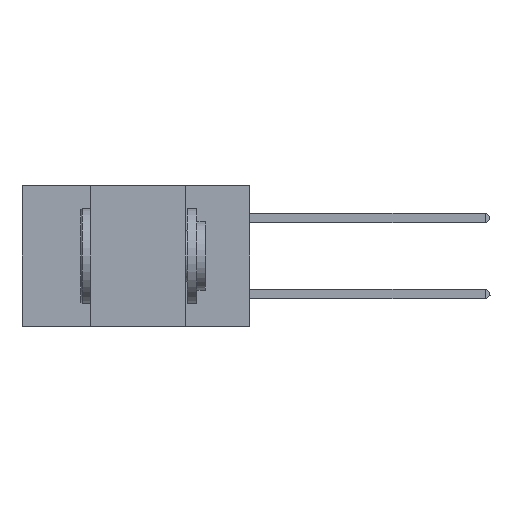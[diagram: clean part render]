
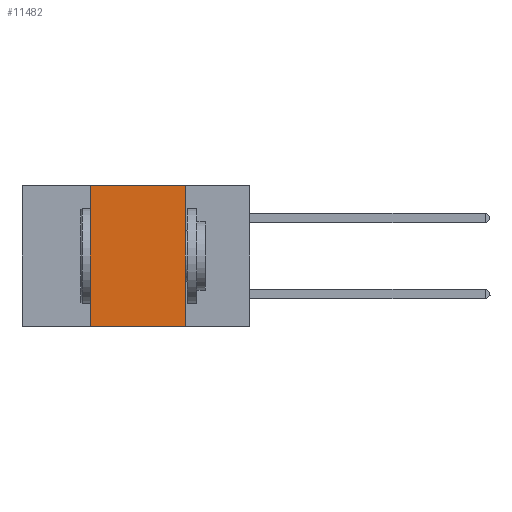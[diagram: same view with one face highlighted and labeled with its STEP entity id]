
A CAD part, left-side view. The second image highlights one B-rep face of the part: STEP entity #11482.
In plain terms, the highlighted planar face has unit normal (-1, 0, 0).
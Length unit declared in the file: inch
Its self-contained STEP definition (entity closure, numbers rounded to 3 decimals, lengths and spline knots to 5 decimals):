
#1263 = DIRECTION ( 'NONE',  ( 0., -1., 0. ) ) ;
#2690 = LINE ( 'NONE', #13811, #7510 ) ;
#3364 = ORIENTED_EDGE ( 'NONE', *, *, #7947, .F. ) ;
#3888 = VERTEX_POINT ( 'NONE', #11872 ) ;
#3892 = LINE ( 'NONE', #11522, #5864 ) ;
#4083 = LINE ( 'NONE', #10778, #4418 ) ;
#4418 = VECTOR ( 'NONE', #17061, 39.37008 ) ;
#5084 = EDGE_CURVE ( 'NONE', #7061, #24200, #3892, .T. ) ;
#5864 = VECTOR ( 'NONE', #1263, 39.37008 ) ;
#6577 = AXIS2_PLACEMENT_3D ( 'NONE', #9366, #25647, #23700 ) ;
#7061 = VERTEX_POINT ( 'NONE', #21695 ) ;
#7291 = ORIENTED_EDGE ( 'NONE', *, *, #5084, .T. ) ;
#7510 = VECTOR ( 'NONE', #16048, 39.37008 ) ;
#7820 = EDGE_CURVE ( 'NONE', #10284, #3888, #2690, .T. ) ;
#7947 = EDGE_CURVE ( 'NONE', #7061, #10284, #12019, .T. ) ;
#9285 = PLANE ( 'NONE',  #6577 ) ;
#9366 = CARTESIAN_POINT ( 'NONE',  ( 0., 0.6, 0. ) ) ;
#10284 = VERTEX_POINT ( 'NONE', #13207 ) ;
#10467 = ORIENTED_EDGE ( 'NONE', *, *, #7820, .F. ) ;
#10729 = EDGE_CURVE ( 'NONE', #3888, #24200, #4083, .T. ) ;
#10778 = CARTESIAN_POINT ( 'NONE',  ( 0., 0.17, 0. ) ) ;
#11482 = ADVANCED_FACE ( 'NONE', ( #15931 ), #9285, .F. ) ;
#11522 = CARTESIAN_POINT ( 'NONE',  ( 0., 0.6, -0.37 ) ) ;
#11872 = CARTESIAN_POINT ( 'NONE',  ( 0., 0.17, 0. ) ) ;
#12019 = LINE ( 'NONE', #14170, #20092 ) ;
#12387 = DIRECTION ( 'NONE',  ( 0., 0., 1. ) ) ;
#12633 = EDGE_LOOP ( 'NONE', ( #26309, #10467, #3364, #7291 ) ) ;
#13207 = CARTESIAN_POINT ( 'NONE',  ( 0., 0.42, 0. ) ) ;
#13811 = CARTESIAN_POINT ( 'NONE',  ( 0., 0.6, 0. ) ) ;
#14170 = CARTESIAN_POINT ( 'NONE',  ( 0., 0.42, 0. ) ) ;
#15931 = FACE_OUTER_BOUND ( 'NONE', #12633, .T. ) ;
#16048 = DIRECTION ( 'NONE',  ( 0., -1., 0. ) ) ;
#17061 = DIRECTION ( 'NONE',  ( 0., 0., -1. ) ) ;
#20092 = VECTOR ( 'NONE', #12387, 39.37008 ) ;
#21695 = CARTESIAN_POINT ( 'NONE',  ( 0., 0.42, -0.37 ) ) ;
#22595 = CARTESIAN_POINT ( 'NONE',  ( 0., 0.17, -0.37 ) ) ;
#23700 = DIRECTION ( 'NONE',  ( 0., 0., -1. ) ) ;
#24200 = VERTEX_POINT ( 'NONE', #22595 ) ;
#25647 = DIRECTION ( 'NONE',  ( 1., 0., 0. ) ) ;
#26309 = ORIENTED_EDGE ( 'NONE', *, *, #10729, .F. ) ;
